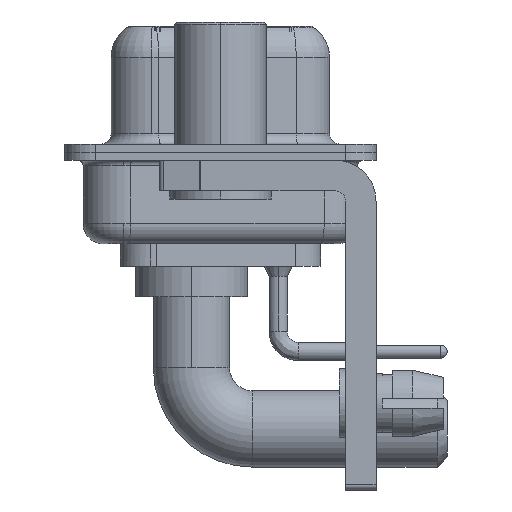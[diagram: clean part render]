
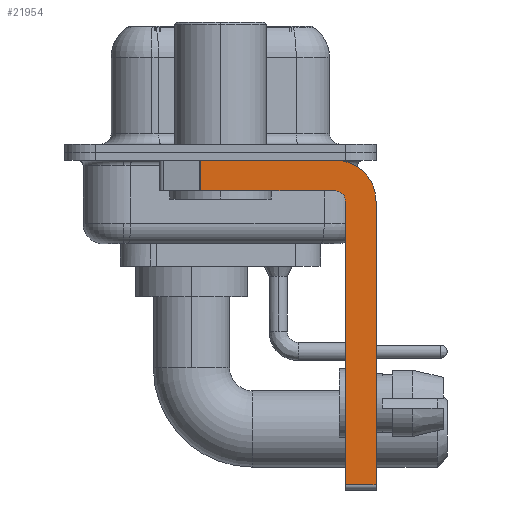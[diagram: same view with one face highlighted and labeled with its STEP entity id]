
A CAD part, left-side view. The second image highlights one B-rep face of the part: STEP entity #21954.
In plain terms, the highlighted planar face has unit normal (-1, 0, 0).
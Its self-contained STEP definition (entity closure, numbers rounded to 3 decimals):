
#577 = LINE ( 'NONE', #12470, #18295 ) ;
#1333 = ORIENTED_EDGE ( 'NONE', *, *, #4100, .F. ) ;
#1394 = CARTESIAN_POINT ( 'NONE',  ( -2.9, -5.65, -2.4 ) ) ;
#2291 = EDGE_CURVE ( 'NONE', #18702, #12214, #22968, .T. ) ;
#2565 = ORIENTED_EDGE ( 'NONE', *, *, #24300, .T. ) ;
#2653 = AXIS2_PLACEMENT_3D ( 'NONE', #1394, #5280, #22451 ) ;
#3052 = VERTEX_POINT ( 'NONE', #17503 ) ;
#3743 = CARTESIAN_POINT ( 'NONE',  ( -2.9, -5.65, -2.4 ) ) ;
#3828 = LINE ( 'NONE', #4070, #20305 ) ;
#3964 = ORIENTED_EDGE ( 'NONE', *, *, #2291, .F. ) ;
#4070 = CARTESIAN_POINT ( 'NONE',  ( -2.9, -5.65, -16.35 ) ) ;
#4100 = EDGE_CURVE ( 'NONE', #11651, #3052, #22594, .T. ) ;
#4111 = VECTOR ( 'NONE', #17351, 1000. ) ;
#4154 = CARTESIAN_POINT ( 'NONE',  ( -2.9, -5.65, -2.4 ) ) ;
#4907 = CARTESIAN_POINT ( 'NONE',  ( -2.9, -6.15, -2.4 ) ) ;
#4999 = CARTESIAN_POINT ( 'NONE',  ( -2.9, -7.65, -2.4 ) ) ;
#5280 = DIRECTION ( 'NONE',  ( 1., 0., 0. ) ) ;
#5737 = EDGE_LOOP ( 'NONE', ( #16204, #13850, #8179, #1333, #18245, #2565, #3964, #14797 ) ) ;
#6282 = DIRECTION ( 'NONE',  ( 0., 0., 1. ) ) ;
#6657 = EDGE_CURVE ( 'NONE', #9863, #18702, #7917, .T. ) ;
#7007 = CARTESIAN_POINT ( 'NONE',  ( -2.9, 3., -0.4 ) ) ;
#7504 = VECTOR ( 'NONE', #22812, 1000. ) ;
#7917 = CIRCLE ( 'NONE', #22727, 2. ) ;
#8179 = ORIENTED_EDGE ( 'NONE', *, *, #12456, .F. ) ;
#8202 = DIRECTION ( 'NONE',  ( 0., 1., 0. ) ) ;
#8637 = LINE ( 'NONE', #7007, #9690 ) ;
#9308 = LINE ( 'NONE', #15088, #17645 ) ;
#9690 = VECTOR ( 'NONE', #12293, 1000. ) ;
#9863 = VERTEX_POINT ( 'NONE', #16602 ) ;
#11572 = CARTESIAN_POINT ( 'NONE',  ( -2.9, 0.978, -1.9 ) ) ;
#11651 = VERTEX_POINT ( 'NONE', #4907 ) ;
#11662 = VERTEX_POINT ( 'NONE', #18451 ) ;
#11806 = DIRECTION ( 'NONE',  ( -1., 0., 0. ) ) ;
#12214 = VERTEX_POINT ( 'NONE', #21371 ) ;
#12293 = DIRECTION ( 'NONE',  ( 0., -1., 0. ) ) ;
#12456 = EDGE_CURVE ( 'NONE', #3052, #15141, #577, .T. ) ;
#12470 = CARTESIAN_POINT ( 'NONE',  ( -2.9, -5.65, -1.9 ) ) ;
#13152 = EDGE_CURVE ( 'NONE', #11662, #11651, #24685, .T. ) ;
#13259 = DIRECTION ( 'NONE',  ( 1., 0., 0. ) ) ;
#13850 = ORIENTED_EDGE ( 'NONE', *, *, #17627, .T. ) ;
#14797 = ORIENTED_EDGE ( 'NONE', *, *, #6657, .F. ) ;
#15088 = CARTESIAN_POINT ( 'NONE',  ( -2.9, 0.978, -1.9 ) ) ;
#15141 = VERTEX_POINT ( 'NONE', #11572 ) ;
#16204 = ORIENTED_EDGE ( 'NONE', *, *, #20183, .F. ) ;
#16489 = VERTEX_POINT ( 'NONE', #17105 ) ;
#16602 = CARTESIAN_POINT ( 'NONE',  ( -2.9, -5.65, -0.4 ) ) ;
#16954 = CARTESIAN_POINT ( 'NONE',  ( -2.9, -6.15, -16.6 ) ) ;
#16981 = DIRECTION ( 'NONE',  ( 0., 0., -1. ) ) ;
#17105 = CARTESIAN_POINT ( 'NONE',  ( -2.9, 0.978, -0.4 ) ) ;
#17351 = DIRECTION ( 'NONE',  ( 0., 0., -1. ) ) ;
#17503 = CARTESIAN_POINT ( 'NONE',  ( -2.9, -5.65, -1.9 ) ) ;
#17627 = EDGE_CURVE ( 'NONE', #16489, #15141, #9308, .T. ) ;
#17645 = VECTOR ( 'NONE', #16981, 1000. ) ;
#18245 = ORIENTED_EDGE ( 'NONE', *, *, #13152, .F. ) ;
#18295 = VECTOR ( 'NONE', #8202, 1000. ) ;
#18451 = CARTESIAN_POINT ( 'NONE',  ( -2.9, -6.15, -16.35 ) ) ;
#18702 = VERTEX_POINT ( 'NONE', #4999 ) ;
#20183 = EDGE_CURVE ( 'NONE', #16489, #9863, #8637, .T. ) ;
#20305 = VECTOR ( 'NONE', #23100, 1000. ) ;
#21093 = CARTESIAN_POINT ( 'NONE',  ( -2.9, -7.65, -2.4 ) ) ;
#21371 = CARTESIAN_POINT ( 'NONE',  ( -2.9, -7.65, -16.35 ) ) ;
#21954 = ADVANCED_FACE ( 'NONE', ( #22330 ), #24689, .F. ) ;
#22330 = FACE_OUTER_BOUND ( 'NONE', #5737, .T. ) ;
#22451 = DIRECTION ( 'NONE',  ( 0., 0., -1. ) ) ;
#22594 = CIRCLE ( 'NONE', #23372, 0.5 ) ;
#22727 = AXIS2_PLACEMENT_3D ( 'NONE', #3743, #13259, #24516 ) ;
#22812 = DIRECTION ( 'NONE',  ( 0., 0., 1. ) ) ;
#22968 = LINE ( 'NONE', #21093, #4111 ) ;
#23100 = DIRECTION ( 'NONE',  ( 0., -1., 0. ) ) ;
#23372 = AXIS2_PLACEMENT_3D ( 'NONE', #4154, #11806, #6282 ) ;
#24300 = EDGE_CURVE ( 'NONE', #11662, #12214, #3828, .T. ) ;
#24516 = DIRECTION ( 'NONE',  ( 0., 0., -1. ) ) ;
#24685 = LINE ( 'NONE', #16954, #7504 ) ;
#24689 = PLANE ( 'NONE',  #2653 ) ;
